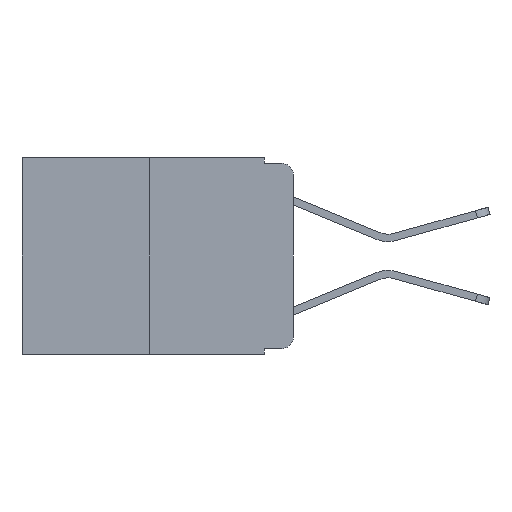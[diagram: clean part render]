
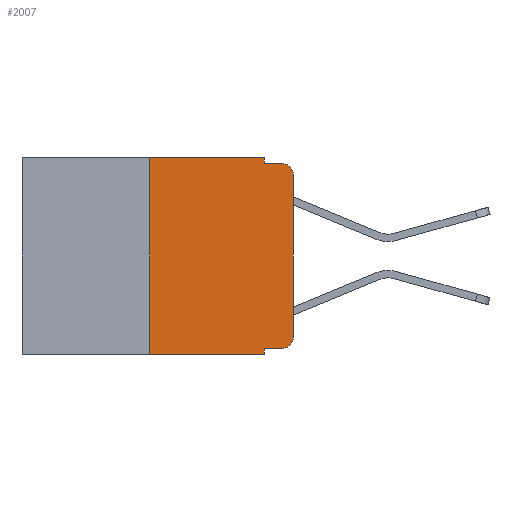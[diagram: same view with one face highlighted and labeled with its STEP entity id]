
A CAD part, left-side view. The second image highlights one B-rep face of the part: STEP entity #2007.
In plain terms, the highlighted planar face has unit normal (-1, 0, 0).
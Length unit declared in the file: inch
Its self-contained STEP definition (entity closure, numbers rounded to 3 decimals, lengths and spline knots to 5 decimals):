
#124 = EDGE_CURVE ( 'NONE', #5621, #3458, #4326, .T. ) ;
#397 = ORIENTED_EDGE ( 'NONE', *, *, #124, .F. ) ;
#721 = LINE ( 'NONE', #17324, #11278 ) ;
#792 = CARTESIAN_POINT ( 'NONE',  ( 0., 0.02, -0.333 ) ) ;
#928 = LINE ( 'NONE', #8222, #15774 ) ;
#1505 = VERTEX_POINT ( 'NONE', #1930 ) ;
#1636 = ORIENTED_EDGE ( 'NONE', *, *, #18025, .F. ) ;
#1930 = CARTESIAN_POINT ( 'NONE',  ( 0., 0.051, -0.343 ) ) ;
#2007 = ADVANCED_FACE ( 'NONE', ( #11763 ), #18249, .F. ) ;
#2327 = VECTOR ( 'NONE', #13148, 39.37008 ) ;
#2788 = CARTESIAN_POINT ( 'NONE',  ( 0., 0.25, 0. ) ) ;
#2953 = DIRECTION ( 'NONE',  ( 0., 0., -1. ) ) ;
#3458 = VERTEX_POINT ( 'NONE', #14152 ) ;
#3674 = CARTESIAN_POINT ( 'NONE',  ( 0., 0., -0.03 ) ) ;
#3753 = VERTEX_POINT ( 'NONE', #8733 ) ;
#4008 = AXIS2_PLACEMENT_3D ( 'NONE', #15302, #6802, #16738 ) ;
#4040 = ORIENTED_EDGE ( 'NONE', *, *, #14698, .T. ) ;
#4326 = LINE ( 'NONE', #12125, #8515 ) ;
#4560 = VERTEX_POINT ( 'NONE', #8416 ) ;
#4658 = VERTEX_POINT ( 'NONE', #10843 ) ;
#4665 = VERTEX_POINT ( 'NONE', #12743 ) ;
#4948 = DIRECTION ( 'NONE',  ( 0., 0., -1. ) ) ;
#5621 = VERTEX_POINT ( 'NONE', #8469 ) ;
#5755 = CARTESIAN_POINT ( 'NONE',  ( 0., 0.02, -0.03 ) ) ;
#5924 = CARTESIAN_POINT ( 'NONE',  ( 0., 0.051, 0. ) ) ;
#5993 = DIRECTION ( 'NONE',  ( -1., 0., 0. ) ) ;
#6078 = ORIENTED_EDGE ( 'NONE', *, *, #14394, .T. ) ;
#6098 = AXIS2_PLACEMENT_3D ( 'NONE', #8364, #10243, #2953 ) ;
#6459 = EDGE_CURVE ( 'NONE', #7169, #16175, #7465, .T. ) ;
#6496 = DIRECTION ( 'NONE',  ( 0., -1., 0. ) ) ;
#6802 = DIRECTION ( 'NONE',  ( -1., 0., 0. ) ) ;
#7169 = VERTEX_POINT ( 'NONE', #3674 ) ;
#7178 = VERTEX_POINT ( 'NONE', #792 ) ;
#7180 = LINE ( 'NONE', #14993, #18082 ) ;
#7342 = DIRECTION ( 'NONE',  ( 0., 0., -1. ) ) ;
#7465 = CIRCLE ( 'NONE', #13112, 0.02 ) ;
#8183 = EDGE_CURVE ( 'NONE', #4560, #1505, #7180, .T. ) ;
#8222 = CARTESIAN_POINT ( 'NONE',  ( 0., 0., 0. ) ) ;
#8298 = EDGE_CURVE ( 'NONE', #7178, #4665, #12903, .T. ) ;
#8364 = CARTESIAN_POINT ( 'NONE',  ( 0., 0.473, 0. ) ) ;
#8416 = CARTESIAN_POINT ( 'NONE',  ( 0., 0.25, -0.343 ) ) ;
#8455 = EDGE_CURVE ( 'NONE', #4560, #3753, #10180, .T. ) ;
#8469 = CARTESIAN_POINT ( 'NONE',  ( 0., 0.051, 0. ) ) ;
#8515 = VECTOR ( 'NONE', #14342, 39.37008 ) ;
#8588 = DIRECTION ( 'NONE',  ( 0., -1., 0. ) ) ;
#8733 = CARTESIAN_POINT ( 'NONE',  ( 0., 0.25, 0. ) ) ;
#8875 = VECTOR ( 'NONE', #8588, 39.37008 ) ;
#8987 = EDGE_LOOP ( 'NONE', ( #6078, #9735, #11439, #397, #11608, #12630, #11103, #1636, #4040, #16579 ) ) ;
#9584 = DIRECTION ( 'NONE',  ( 0., 0., 1. ) ) ;
#9735 = ORIENTED_EDGE ( 'NONE', *, *, #6459, .T. ) ;
#10140 = DIRECTION ( 'NONE',  ( 0., -1., 0. ) ) ;
#10180 = LINE ( 'NONE', #2788, #14504 ) ;
#10243 = DIRECTION ( 'NONE',  ( 1., 0., 0. ) ) ;
#10843 = CARTESIAN_POINT ( 'NONE',  ( 0., 0.051, -0.333 ) ) ;
#11103 = ORIENTED_EDGE ( 'NONE', *, *, #8183, .T. ) ;
#11261 = LINE ( 'NONE', #5924, #14674 ) ;
#11278 = VECTOR ( 'NONE', #10140, 39.37008 ) ;
#11299 = DIRECTION ( 'NONE',  ( 0., 0., 1. ) ) ;
#11347 = CARTESIAN_POINT ( 'NONE',  ( 0., 0.473, 0. ) ) ;
#11439 = ORIENTED_EDGE ( 'NONE', *, *, #16934, .F. ) ;
#11608 = ORIENTED_EDGE ( 'NONE', *, *, #16851, .F. ) ;
#11713 = CARTESIAN_POINT ( 'NONE',  ( 0., 0.051, -0.333 ) ) ;
#11763 = FACE_OUTER_BOUND ( 'NONE', #8987, .T. ) ;
#12125 = CARTESIAN_POINT ( 'NONE',  ( 0., 0.051, 0. ) ) ;
#12630 = ORIENTED_EDGE ( 'NONE', *, *, #8455, .F. ) ;
#12638 = LINE ( 'NONE', #11347, #8875 ) ;
#12743 = CARTESIAN_POINT ( 'NONE',  ( 0., 0., -0.313 ) ) ;
#12903 = CIRCLE ( 'NONE', #4008, 0.02 ) ;
#13112 = AXIS2_PLACEMENT_3D ( 'NONE', #5755, #5993, #4948 ) ;
#13148 = DIRECTION ( 'NONE',  ( 0., -1., 0. ) ) ;
#13745 = LINE ( 'NONE', #11713, #2327 ) ;
#14152 = CARTESIAN_POINT ( 'NONE',  ( 0., 0.051, -0.01 ) ) ;
#14342 = DIRECTION ( 'NONE',  ( 0., 0., -1. ) ) ;
#14394 = EDGE_CURVE ( 'NONE', #4665, #7169, #928, .T. ) ;
#14504 = VECTOR ( 'NONE', #11299, 39.37008 ) ;
#14674 = VECTOR ( 'NONE', #7342, 39.37008 ) ;
#14698 = EDGE_CURVE ( 'NONE', #4658, #7178, #13745, .T. ) ;
#14993 = CARTESIAN_POINT ( 'NONE',  ( 0., 0.473, -0.343 ) ) ;
#15302 = CARTESIAN_POINT ( 'NONE',  ( 0., 0.02, -0.313 ) ) ;
#15774 = VECTOR ( 'NONE', #9584, 39.37008 ) ;
#16175 = VERTEX_POINT ( 'NONE', #16762 ) ;
#16579 = ORIENTED_EDGE ( 'NONE', *, *, #8298, .T. ) ;
#16738 = DIRECTION ( 'NONE',  ( 0., 0., -1. ) ) ;
#16762 = CARTESIAN_POINT ( 'NONE',  ( 0., 0.02, -0.01 ) ) ;
#16851 = EDGE_CURVE ( 'NONE', #3753, #5621, #12638, .T. ) ;
#16934 = EDGE_CURVE ( 'NONE', #3458, #16175, #721, .T. ) ;
#17324 = CARTESIAN_POINT ( 'NONE',  ( 0., 0.051, -0.01 ) ) ;
#18025 = EDGE_CURVE ( 'NONE', #4658, #1505, #11261, .T. ) ;
#18082 = VECTOR ( 'NONE', #6496, 39.37008 ) ;
#18249 = PLANE ( 'NONE',  #6098 ) ;
